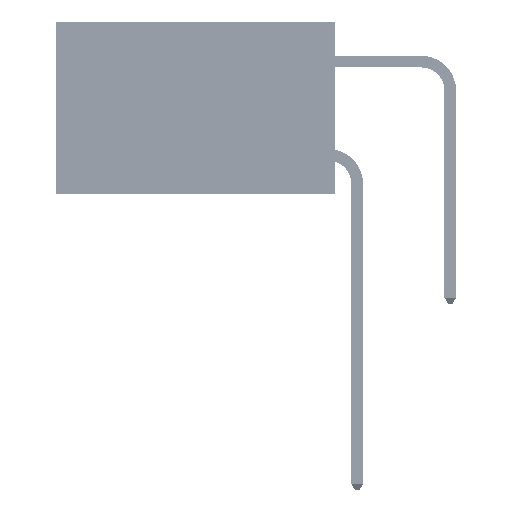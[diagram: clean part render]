
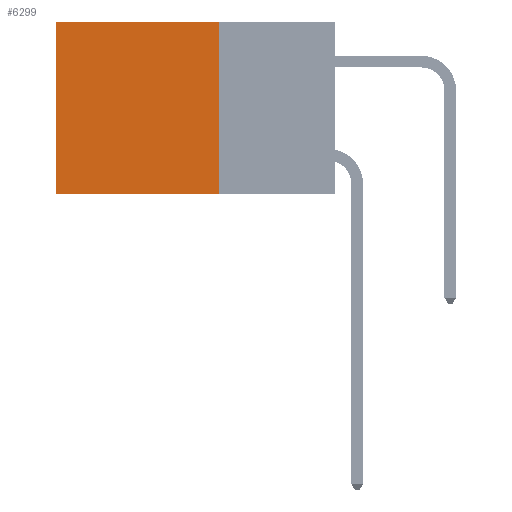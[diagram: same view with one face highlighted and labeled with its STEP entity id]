
A CAD part, left-side view. The second image highlights one B-rep face of the part: STEP entity #6299.
In plain terms, the highlighted planar face has unit normal (-1, 0, 0).
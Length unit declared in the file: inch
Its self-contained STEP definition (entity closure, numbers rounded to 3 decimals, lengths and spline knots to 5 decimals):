
#432 = ORIENTED_EDGE ( 'NONE', *, *, #27753, .F. ) ;
#734 = VERTEX_POINT ( 'NONE', #42546 ) ;
#1283 = EDGE_CURVE ( 'NONE', #27171, #21040, #45296, .T. ) ;
#3194 = DIRECTION ( 'NONE',  ( 0., 1., 0. ) ) ;
#3574 = VECTOR ( 'NONE', #5395, 39.37008 ) ;
#5395 = DIRECTION ( 'NONE',  ( 0., 0., -1. ) ) ;
#6299 = ADVANCED_FACE ( 'NONE', ( #19763 ), #21033, .F. ) ;
#7258 = EDGE_LOOP ( 'NONE', ( #16169, #432, #30739, #10331 ) ) ;
#10331 = ORIENTED_EDGE ( 'NONE', *, *, #32677, .T. ) ;
#12347 = EDGE_CURVE ( 'NONE', #734, #19431, #13168, .T. ) ;
#13168 = LINE ( 'NONE', #33949, #3574 ) ;
#14973 = VECTOR ( 'NONE', #18952, 39.37008 ) ;
#16169 = ORIENTED_EDGE ( 'NONE', *, *, #1283, .T. ) ;
#18952 = DIRECTION ( 'NONE',  ( 0., 1., 0. ) ) ;
#19431 = VERTEX_POINT ( 'NONE', #35634 ) ;
#19576 = CARTESIAN_POINT ( 'NONE',  ( 0.2875, 0.6, -0.37 ) ) ;
#19763 = FACE_OUTER_BOUND ( 'NONE', #7258, .T. ) ;
#21033 = PLANE ( 'NONE',  #21161 ) ;
#21040 = VERTEX_POINT ( 'NONE', #19576 ) ;
#21161 = AXIS2_PLACEMENT_3D ( 'NONE', #31644, #45821, #24612 ) ;
#21201 = CARTESIAN_POINT ( 'NONE',  ( 0.2875, 0.25, 0. ) ) ;
#24253 = VECTOR ( 'NONE', #44983, 39.37008 ) ;
#24612 = DIRECTION ( 'NONE',  ( 0., 0., -1. ) ) ;
#27171 = VERTEX_POINT ( 'NONE', #30114 ) ;
#27753 = EDGE_CURVE ( 'NONE', #19431, #21040, #43374, .T. ) ;
#30114 = CARTESIAN_POINT ( 'NONE',  ( 0.2875, 0.6, 0. ) ) ;
#30739 = ORIENTED_EDGE ( 'NONE', *, *, #12347, .F. ) ;
#31644 = CARTESIAN_POINT ( 'NONE',  ( 0.2875, 0.25, 0. ) ) ;
#32677 = EDGE_CURVE ( 'NONE', #734, #27171, #40733, .T. ) ;
#33949 = CARTESIAN_POINT ( 'NONE',  ( 0.2875, 0.25, 0. ) ) ;
#35634 = CARTESIAN_POINT ( 'NONE',  ( 0.2875, 0.25, -0.37 ) ) ;
#36747 = CARTESIAN_POINT ( 'NONE',  ( 0.2875, 0.25, -0.37 ) ) ;
#39630 = VECTOR ( 'NONE', #3194, 39.37008 ) ;
#40733 = LINE ( 'NONE', #21201, #39630 ) ;
#41405 = CARTESIAN_POINT ( 'NONE',  ( 0.2875, 0.6, 0. ) ) ;
#42546 = CARTESIAN_POINT ( 'NONE',  ( 0.2875, 0.25, 0. ) ) ;
#43374 = LINE ( 'NONE', #36747, #14973 ) ;
#44983 = DIRECTION ( 'NONE',  ( 0., 0., -1. ) ) ;
#45296 = LINE ( 'NONE', #41405, #24253 ) ;
#45821 = DIRECTION ( 'NONE',  ( 1., 0., 0. ) ) ;
